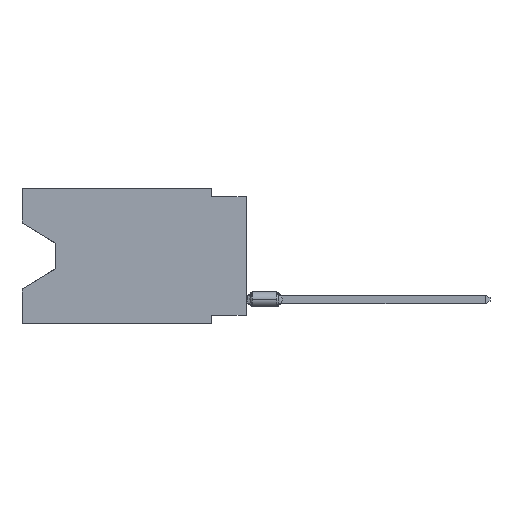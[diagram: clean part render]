
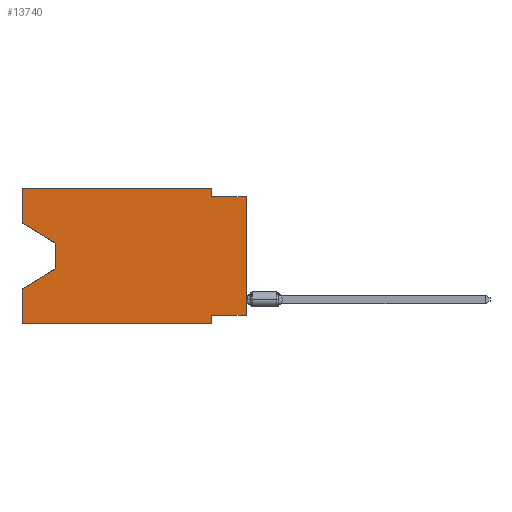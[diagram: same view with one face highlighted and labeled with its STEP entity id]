
A CAD part, left-side view. The second image highlights one B-rep face of the part: STEP entity #13740.
In plain terms, the highlighted planar face has unit normal (-1, 0, 0).
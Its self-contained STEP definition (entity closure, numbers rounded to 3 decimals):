
#228 = DIRECTION ( 'NONE',  ( 0., -1., 0. ) ) ;
#312 = CARTESIAN_POINT ( 'NONE',  ( 0., 16.383, -9.906 ) ) ;
#636 = LINE ( 'NONE', #27024, #18513 ) ;
#962 = CARTESIAN_POINT ( 'NONE',  ( 0., 13.97, -4.013 ) ) ;
#1950 = DIRECTION ( 'NONE',  ( 0., 0., 1. ) ) ;
#2114 = VERTEX_POINT ( 'NONE', #8443 ) ;
#2231 = VECTOR ( 'NONE', #1950, 1000. ) ;
#2588 = DIRECTION ( 'NONE',  ( 0., -1., 0. ) ) ;
#3043 = EDGE_LOOP ( 'NONE', ( #15115, #26303, #5485, #6239, #11895, #20377, #31172, #24128, #27928, #11043, #17859, #5750 ) ) ;
#3276 = CARTESIAN_POINT ( 'NONE',  ( 0., 0., 0. ) ) ;
#4405 = PLANE ( 'NONE',  #12174 ) ;
#4455 = CARTESIAN_POINT ( 'NONE',  ( 0., 0., -9.271 ) ) ;
#5185 = DIRECTION ( 'NONE',  ( 0., 0., -1. ) ) ;
#5410 = CARTESIAN_POINT ( 'NONE',  ( 0., 0., -0.635 ) ) ;
#5485 = ORIENTED_EDGE ( 'NONE', *, *, #8837, .T. ) ;
#5547 = DIRECTION ( 'NONE',  ( 0., -0.855, -0.519 ) ) ;
#5750 = ORIENTED_EDGE ( 'NONE', *, *, #20564, .F. ) ;
#5823 = VERTEX_POINT ( 'NONE', #18811 ) ;
#6239 = ORIENTED_EDGE ( 'NONE', *, *, #31005, .F. ) ;
#6335 = LINE ( 'NONE', #8761, #26503 ) ;
#6942 = VERTEX_POINT ( 'NONE', #5410 ) ;
#7246 = EDGE_CURVE ( 'NONE', #31308, #22785, #25262, .T. ) ;
#7425 = EDGE_CURVE ( 'NONE', #30318, #5823, #31612, .T. ) ;
#8443 = CARTESIAN_POINT ( 'NONE',  ( 0., 16.383, -9.906 ) ) ;
#8561 = DIRECTION ( 'NONE',  ( 0., 0., -1. ) ) ;
#8761 = CARTESIAN_POINT ( 'NONE',  ( 0., 0., -0.635 ) ) ;
#8837 = EDGE_CURVE ( 'NONE', #22785, #23330, #19660, .T. ) ;
#9505 = CARTESIAN_POINT ( 'NONE',  ( 0., 0., -9.271 ) ) ;
#10350 = CARTESIAN_POINT ( 'NONE',  ( 0., 16.383, -2.546 ) ) ;
#10446 = VECTOR ( 'NONE', #5547, 1000. ) ;
#10536 = CARTESIAN_POINT ( 'NONE',  ( 0., 2.54, -0.635 ) ) ;
#10964 = VECTOR ( 'NONE', #16590, 1000. ) ;
#11043 = ORIENTED_EDGE ( 'NONE', *, *, #17599, .F. ) ;
#11369 = EDGE_CURVE ( 'NONE', #16445, #31308, #20271, .T. ) ;
#11585 = EDGE_CURVE ( 'NONE', #28175, #6942, #27870, .T. ) ;
#11842 = VERTEX_POINT ( 'NONE', #29457 ) ;
#11895 = ORIENTED_EDGE ( 'NONE', *, *, #14250, .T. ) ;
#11982 = CARTESIAN_POINT ( 'NONE',  ( 0., 16.383, 0. ) ) ;
#12174 = AXIS2_PLACEMENT_3D ( 'NONE', #24303, #31733, #19137 ) ;
#12707 = VECTOR ( 'NONE', #2588, 1000. ) ;
#12813 = CARTESIAN_POINT ( 'NONE',  ( 0., 13.97, -4.013 ) ) ;
#13740 = ADVANCED_FACE ( 'NONE', ( #21549 ), #4405, .F. ) ;
#14250 = EDGE_CURVE ( 'NONE', #2114, #11842, #17152, .T. ) ;
#14587 = CARTESIAN_POINT ( 'NONE',  ( 0., 16.383, 0. ) ) ;
#15115 = ORIENTED_EDGE ( 'NONE', *, *, #11369, .T. ) ;
#16445 = VERTEX_POINT ( 'NONE', #10350 ) ;
#16525 = EDGE_CURVE ( 'NONE', #25697, #11842, #30225, .T. ) ;
#16590 = DIRECTION ( 'NONE',  ( 0., 1., 0. ) ) ;
#16855 = VECTOR ( 'NONE', #24605, 1000. ) ;
#17152 = LINE ( 'NONE', #312, #12707 ) ;
#17559 = CARTESIAN_POINT ( 'NONE',  ( 0., 13.97, -5.893 ) ) ;
#17599 = EDGE_CURVE ( 'NONE', #5823, #28559, #636, .T. ) ;
#17859 = ORIENTED_EDGE ( 'NONE', *, *, #7425, .F. ) ;
#18472 = DIRECTION ( 'NONE',  ( 0., -1., 0. ) ) ;
#18513 = VECTOR ( 'NONE', #5185, 1000. ) ;
#18811 = CARTESIAN_POINT ( 'NONE',  ( 0., 2.54, 0. ) ) ;
#19137 = DIRECTION ( 'NONE',  ( 0., 0., -1. ) ) ;
#19660 = LINE ( 'NONE', #17559, #20676 ) ;
#19760 = LINE ( 'NONE', #14587, #16855 ) ;
#20271 = LINE ( 'NONE', #27701, #10446 ) ;
#20377 = ORIENTED_EDGE ( 'NONE', *, *, #16525, .F. ) ;
#20381 = CARTESIAN_POINT ( 'NONE',  ( 0., 2.54, -9.906 ) ) ;
#20564 = EDGE_CURVE ( 'NONE', #16445, #30318, #19760, .T. ) ;
#20595 = DIRECTION ( 'NONE',  ( 0., 0., 1. ) ) ;
#20604 = VECTOR ( 'NONE', #228, 1000. ) ;
#20676 = VECTOR ( 'NONE', #25140, 1000. ) ;
#21292 = VECTOR ( 'NONE', #20595, 1000. ) ;
#21549 = FACE_OUTER_BOUND ( 'NONE', #3043, .T. ) ;
#21943 = VECTOR ( 'NONE', #8561, 1000. ) ;
#22324 = CARTESIAN_POINT ( 'NONE',  ( 0., 16.383, -7.36 ) ) ;
#22391 = CARTESIAN_POINT ( 'NONE',  ( 0., 16.383, 0. ) ) ;
#22542 = CARTESIAN_POINT ( 'NONE',  ( 0., 2.54, -9.271 ) ) ;
#22785 = VERTEX_POINT ( 'NONE', #25949 ) ;
#22828 = DIRECTION ( 'NONE',  ( 0., 0., -1. ) ) ;
#23330 = VERTEX_POINT ( 'NONE', #22324 ) ;
#24128 = ORIENTED_EDGE ( 'NONE', *, *, #11585, .T. ) ;
#24303 = CARTESIAN_POINT ( 'NONE',  ( 0., 16.383, 0. ) ) ;
#24605 = DIRECTION ( 'NONE',  ( 0., 0., 1. ) ) ;
#25140 = DIRECTION ( 'NONE',  ( 0., 0.855, -0.519 ) ) ;
#25262 = LINE ( 'NONE', #12813, #27289 ) ;
#25697 = VERTEX_POINT ( 'NONE', #22542 ) ;
#25949 = CARTESIAN_POINT ( 'NONE',  ( 0., 13.97, -5.893 ) ) ;
#25979 = LINE ( 'NONE', #4455, #10964 ) ;
#26177 = CARTESIAN_POINT ( 'NONE',  ( 0., 16.383, 0. ) ) ;
#26303 = ORIENTED_EDGE ( 'NONE', *, *, #7246, .T. ) ;
#26503 = VECTOR ( 'NONE', #18472, 1000. ) ;
#27024 = CARTESIAN_POINT ( 'NONE',  ( 0., 2.54, 0. ) ) ;
#27289 = VECTOR ( 'NONE', #22828, 1000. ) ;
#27701 = CARTESIAN_POINT ( 'NONE',  ( 0., 16.383, -2.546 ) ) ;
#27870 = LINE ( 'NONE', #3276, #21292 ) ;
#27928 = ORIENTED_EDGE ( 'NONE', *, *, #30789, .F. ) ;
#28175 = VERTEX_POINT ( 'NONE', #9505 ) ;
#28559 = VERTEX_POINT ( 'NONE', #10536 ) ;
#29447 = LINE ( 'NONE', #11982, #2231 ) ;
#29457 = CARTESIAN_POINT ( 'NONE',  ( 0., 2.54, -9.906 ) ) ;
#29541 = EDGE_CURVE ( 'NONE', #28175, #25697, #25979, .T. ) ;
#30225 = LINE ( 'NONE', #20381, #21943 ) ;
#30318 = VERTEX_POINT ( 'NONE', #26177 ) ;
#30789 = EDGE_CURVE ( 'NONE', #28559, #6942, #6335, .T. ) ;
#31005 = EDGE_CURVE ( 'NONE', #2114, #23330, #29447, .T. ) ;
#31172 = ORIENTED_EDGE ( 'NONE', *, *, #29541, .F. ) ;
#31308 = VERTEX_POINT ( 'NONE', #962 ) ;
#31612 = LINE ( 'NONE', #22391, #20604 ) ;
#31733 = DIRECTION ( 'NONE',  ( 1., 0., 0. ) ) ;
